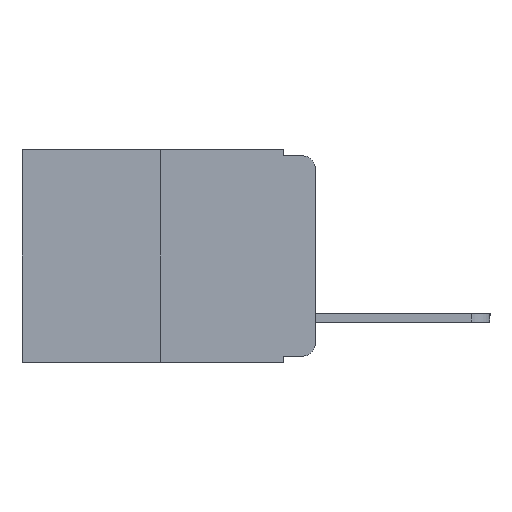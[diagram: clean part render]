
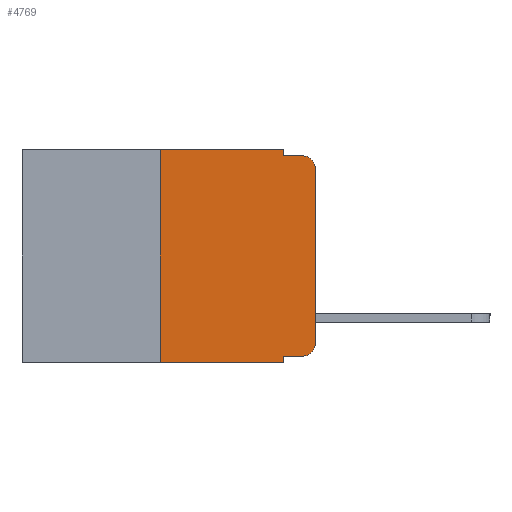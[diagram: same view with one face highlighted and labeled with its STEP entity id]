
A CAD part, left-side view. The second image highlights one B-rep face of the part: STEP entity #4769.
In plain terms, the highlighted planar face has unit normal (-1, 0, 0).
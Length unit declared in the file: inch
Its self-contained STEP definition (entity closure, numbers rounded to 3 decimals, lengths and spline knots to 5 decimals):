
#41 = EDGE_CURVE ( 'NONE', #3082, #7058, #7322, .T. ) ;
#1018 = DIRECTION ( 'NONE',  ( 0., -1., 0. ) ) ;
#1070 = LINE ( 'NONE', #11641, #3502 ) ;
#1099 = EDGE_CURVE ( 'NONE', #8707, #2847, #10633, .T. ) ;
#1254 = CARTESIAN_POINT ( 'NONE',  ( 0., 0.051, -0.333 ) ) ;
#1545 = VERTEX_POINT ( 'NONE', #3608 ) ;
#1880 = CARTESIAN_POINT ( 'NONE',  ( 0., 0., 0. ) ) ;
#1936 = VECTOR ( 'NONE', #3875, 39.37008 ) ;
#2076 = VECTOR ( 'NONE', #5503, 39.37008 ) ;
#2201 = CARTESIAN_POINT ( 'NONE',  ( 0., 0., -0.03 ) ) ;
#2276 = VECTOR ( 'NONE', #11403, 39.37008 ) ;
#2578 = LINE ( 'NONE', #1880, #1936 ) ;
#2654 = ORIENTED_EDGE ( 'NONE', *, *, #3096, .F. ) ;
#2698 = CARTESIAN_POINT ( 'NONE',  ( 0., 0.25, -0.343 ) ) ;
#2767 = CARTESIAN_POINT ( 'NONE',  ( 0., 0., -0.313 ) ) ;
#2799 = ORIENTED_EDGE ( 'NONE', *, *, #11099, .T. ) ;
#2847 = VERTEX_POINT ( 'NONE', #9321 ) ;
#2957 = PLANE ( 'NONE',  #7391 ) ;
#3082 = VERTEX_POINT ( 'NONE', #2201 ) ;
#3096 = EDGE_CURVE ( 'NONE', #10500, #1545, #8956, .T. ) ;
#3481 = VERTEX_POINT ( 'NONE', #7776 ) ;
#3502 = VECTOR ( 'NONE', #6798, 39.37008 ) ;
#3608 = CARTESIAN_POINT ( 'NONE',  ( 0., 0.051, 0. ) ) ;
#3875 = DIRECTION ( 'NONE',  ( 0., 0., 1. ) ) ;
#4069 = ORIENTED_EDGE ( 'NONE', *, *, #1099, .T. ) ;
#4142 = CIRCLE ( 'NONE', #9599, 0.02 ) ;
#4204 = DIRECTION ( 'NONE',  ( -1., 0., 0. ) ) ;
#4299 = VERTEX_POINT ( 'NONE', #2767 ) ;
#4474 = LINE ( 'NONE', #12333, #2076 ) ;
#4576 = CARTESIAN_POINT ( 'NONE',  ( 0., 0.02, -0.01 ) ) ;
#4710 = CARTESIAN_POINT ( 'NONE',  ( 0., 0.02, -0.03 ) ) ;
#4769 = ADVANCED_FACE ( 'NONE', ( #10267 ), #2957, .F. ) ;
#4799 = CARTESIAN_POINT ( 'NONE',  ( 0., 0.473, 0. ) ) ;
#5238 = ORIENTED_EDGE ( 'NONE', *, *, #10434, .F. ) ;
#5503 = DIRECTION ( 'NONE',  ( 0., -1., 0. ) ) ;
#5683 = DIRECTION ( 'NONE',  ( -1., 0., 0. ) ) ;
#6402 = EDGE_LOOP ( 'NONE', ( #7501, #12609, #10084, #10354, #2654, #5238, #4069, #7957, #2799, #10483 ) ) ;
#6683 = CARTESIAN_POINT ( 'NONE',  ( 0., 0.25, 0. ) ) ;
#6798 = DIRECTION ( 'NONE',  ( 0., -1., 0. ) ) ;
#6945 = VECTOR ( 'NONE', #9744, 39.37008 ) ;
#7058 = VERTEX_POINT ( 'NONE', #4576 ) ;
#7322 = CIRCLE ( 'NONE', #9239, 0.02 ) ;
#7391 = AXIS2_PLACEMENT_3D ( 'NONE', #4799, #11699, #11632 ) ;
#7501 = ORIENTED_EDGE ( 'NONE', *, *, #11245, .T. ) ;
#7582 = CARTESIAN_POINT ( 'NONE',  ( 0., 0.25, 0. ) ) ;
#7713 = CARTESIAN_POINT ( 'NONE',  ( 0., 0.051, 0. ) ) ;
#7776 = CARTESIAN_POINT ( 'NONE',  ( 0., 0.02, -0.333 ) ) ;
#7957 = ORIENTED_EDGE ( 'NONE', *, *, #8539, .F. ) ;
#7976 = VERTEX_POINT ( 'NONE', #1254 ) ;
#8107 = VECTOR ( 'NONE', #8182, 39.37008 ) ;
#8169 = VERTEX_POINT ( 'NONE', #10471 ) ;
#8182 = DIRECTION ( 'NONE',  ( 0., -1., 0. ) ) ;
#8532 = LINE ( 'NONE', #7713, #10766 ) ;
#8539 = EDGE_CURVE ( 'NONE', #7976, #2847, #8532, .T. ) ;
#8680 = DIRECTION ( 'NONE',  ( 0., 0., -1. ) ) ;
#8707 = VERTEX_POINT ( 'NONE', #2698 ) ;
#8762 = CARTESIAN_POINT ( 'NONE',  ( 0., 0.051, 0. ) ) ;
#8847 = CARTESIAN_POINT ( 'NONE',  ( 0., 0.473, 0. ) ) ;
#8956 = LINE ( 'NONE', #8847, #12368 ) ;
#9239 = AXIS2_PLACEMENT_3D ( 'NONE', #4710, #5683, #13001 ) ;
#9321 = CARTESIAN_POINT ( 'NONE',  ( 0., 0.051, -0.343 ) ) ;
#9599 = AXIS2_PLACEMENT_3D ( 'NONE', #10217, #4204, #11163 ) ;
#9744 = DIRECTION ( 'NONE',  ( 0., 0., -1. ) ) ;
#10084 = ORIENTED_EDGE ( 'NONE', *, *, #12499, .F. ) ;
#10217 = CARTESIAN_POINT ( 'NONE',  ( 0., 0.02, -0.313 ) ) ;
#10267 = FACE_OUTER_BOUND ( 'NONE', #6402, .T. ) ;
#10354 = ORIENTED_EDGE ( 'NONE', *, *, #11080, .F. ) ;
#10434 = EDGE_CURVE ( 'NONE', #8707, #10500, #12835, .T. ) ;
#10471 = CARTESIAN_POINT ( 'NONE',  ( 0., 0.051, -0.01 ) ) ;
#10483 = ORIENTED_EDGE ( 'NONE', *, *, #12986, .T. ) ;
#10500 = VERTEX_POINT ( 'NONE', #6683 ) ;
#10633 = LINE ( 'NONE', #12768, #8107 ) ;
#10766 = VECTOR ( 'NONE', #8680, 39.37008 ) ;
#11080 = EDGE_CURVE ( 'NONE', #1545, #8169, #11792, .T. ) ;
#11099 = EDGE_CURVE ( 'NONE', #7976, #3481, #1070, .T. ) ;
#11163 = DIRECTION ( 'NONE',  ( 0., 0., -1. ) ) ;
#11245 = EDGE_CURVE ( 'NONE', #4299, #3082, #2578, .T. ) ;
#11403 = DIRECTION ( 'NONE',  ( 0., 0., 1. ) ) ;
#11632 = DIRECTION ( 'NONE',  ( 0., 0., -1. ) ) ;
#11641 = CARTESIAN_POINT ( 'NONE',  ( 0., 0.051, -0.333 ) ) ;
#11699 = DIRECTION ( 'NONE',  ( 1., 0., 0. ) ) ;
#11792 = LINE ( 'NONE', #8762, #6945 ) ;
#12333 = CARTESIAN_POINT ( 'NONE',  ( 0., 0.051, -0.01 ) ) ;
#12368 = VECTOR ( 'NONE', #1018, 39.37008 ) ;
#12499 = EDGE_CURVE ( 'NONE', #8169, #7058, #4474, .T. ) ;
#12609 = ORIENTED_EDGE ( 'NONE', *, *, #41, .T. ) ;
#12768 = CARTESIAN_POINT ( 'NONE',  ( 0., 0.473, -0.343 ) ) ;
#12835 = LINE ( 'NONE', #7582, #2276 ) ;
#12986 = EDGE_CURVE ( 'NONE', #3481, #4299, #4142, .T. ) ;
#13001 = DIRECTION ( 'NONE',  ( 0., 0., -1. ) ) ;
